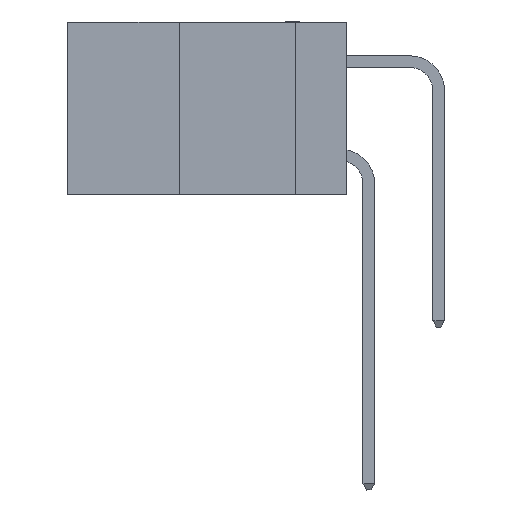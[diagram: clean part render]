
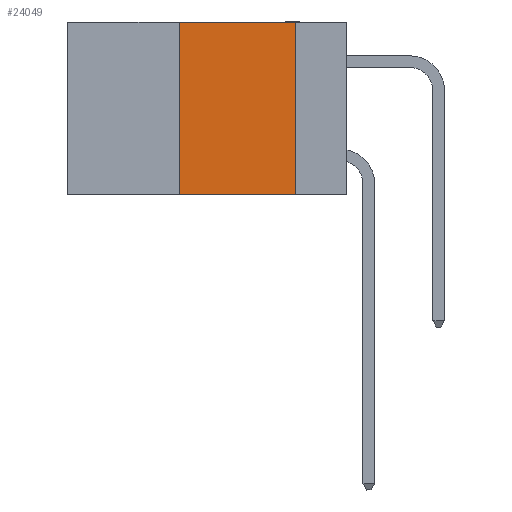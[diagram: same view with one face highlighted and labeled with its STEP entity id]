
A CAD part, left-side view. The second image highlights one B-rep face of the part: STEP entity #24049.
In plain terms, the highlighted planar face has unit normal (-1, 0, 0).
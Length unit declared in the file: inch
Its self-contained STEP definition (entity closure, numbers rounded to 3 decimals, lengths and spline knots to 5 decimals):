
#205 = EDGE_LOOP ( 'NONE', ( #29305, #18412, #14927, #4116 ) ) ;
#1586 = LINE ( 'NONE', #23734, #31905 ) ;
#4116 = ORIENTED_EDGE ( 'NONE', *, *, #12070, .T. ) ;
#4210 = CARTESIAN_POINT ( 'NONE',  ( 0., 0.6, 0. ) ) ;
#4751 = PLANE ( 'NONE',  #35369 ) ;
#6801 = DIRECTION ( 'NONE',  ( 0., 0., 1. ) ) ;
#8803 = LINE ( 'NONE', #33741, #34515 ) ;
#9924 = CARTESIAN_POINT ( 'NONE',  ( 0., 0.36, 0. ) ) ;
#10234 = DIRECTION ( 'NONE',  ( 0., -1., 0. ) ) ;
#10637 = EDGE_CURVE ( 'NONE', #35872, #28502, #8803, .T. ) ;
#11976 = VERTEX_POINT ( 'NONE', #28932 ) ;
#12070 = EDGE_CURVE ( 'NONE', #11976, #24775, #1586, .T. ) ;
#13768 = CARTESIAN_POINT ( 'NONE',  ( 0., 0.11, 0. ) ) ;
#14927 = ORIENTED_EDGE ( 'NONE', *, *, #33527, .F. ) ;
#15470 = LINE ( 'NONE', #9924, #22704 ) ;
#16014 = DIRECTION ( 'NONE',  ( 0., 0., -1. ) ) ;
#18412 = ORIENTED_EDGE ( 'NONE', *, *, #10637, .F. ) ;
#20054 = DIRECTION ( 'NONE',  ( 0., -1., 0. ) ) ;
#20748 = CARTESIAN_POINT ( 'NONE',  ( 0., 0.36, 0. ) ) ;
#21562 = FACE_OUTER_BOUND ( 'NONE', #205, .T. ) ;
#22704 = VECTOR ( 'NONE', #6801, 39.37008 ) ;
#22811 = CARTESIAN_POINT ( 'NONE',  ( 0., 0.11, -0.37 ) ) ;
#23734 = CARTESIAN_POINT ( 'NONE',  ( 0., 0.6, -0.37 ) ) ;
#23844 = VECTOR ( 'NONE', #34120, 39.37008 ) ;
#24049 = ADVANCED_FACE ( 'NONE', ( #21562 ), #4751, .F. ) ;
#24775 = VERTEX_POINT ( 'NONE', #22811 ) ;
#25457 = LINE ( 'NONE', #25984, #23844 ) ;
#25984 = CARTESIAN_POINT ( 'NONE',  ( 0., 0.11, 0. ) ) ;
#26736 = DIRECTION ( 'NONE',  ( 1., 0., 0. ) ) ;
#26884 = EDGE_CURVE ( 'NONE', #28502, #24775, #25457, .T. ) ;
#28502 = VERTEX_POINT ( 'NONE', #13768 ) ;
#28932 = CARTESIAN_POINT ( 'NONE',  ( 0., 0.36, -0.37 ) ) ;
#29305 = ORIENTED_EDGE ( 'NONE', *, *, #26884, .F. ) ;
#31905 = VECTOR ( 'NONE', #10234, 39.37008 ) ;
#33527 = EDGE_CURVE ( 'NONE', #11976, #35872, #15470, .T. ) ;
#33741 = CARTESIAN_POINT ( 'NONE',  ( 0., 0.6, 0. ) ) ;
#34120 = DIRECTION ( 'NONE',  ( 0., 0., -1. ) ) ;
#34515 = VECTOR ( 'NONE', #20054, 39.37008 ) ;
#35369 = AXIS2_PLACEMENT_3D ( 'NONE', #4210, #26736, #16014 ) ;
#35872 = VERTEX_POINT ( 'NONE', #20748 ) ;
